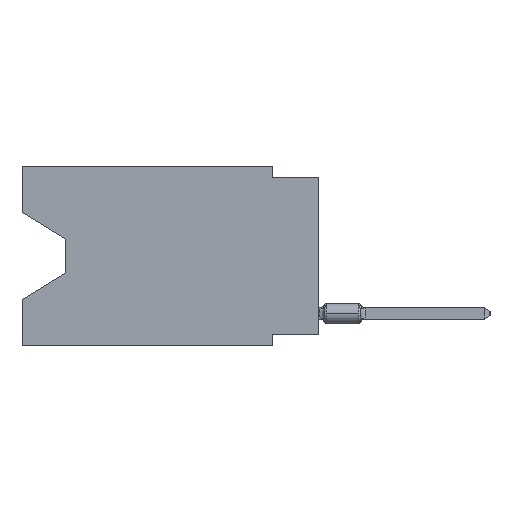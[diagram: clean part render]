
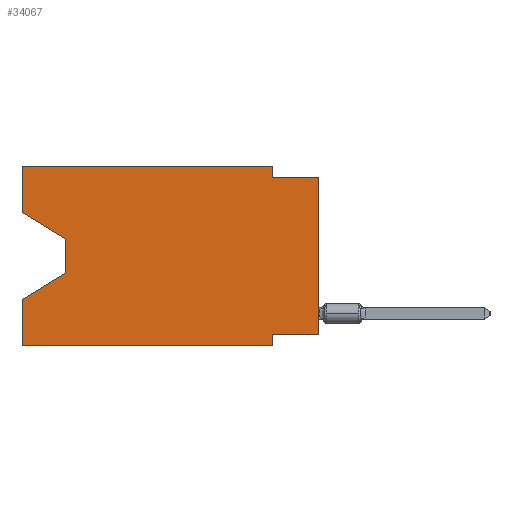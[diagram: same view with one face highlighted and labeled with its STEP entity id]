
A CAD part, left-side view. The second image highlights one B-rep face of the part: STEP entity #34067.
In plain terms, the highlighted planar face has unit normal (-1, 0, 0).
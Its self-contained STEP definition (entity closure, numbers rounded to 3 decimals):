
#341 = CARTESIAN_POINT ( 'NONE',  ( 0., 16.383, 0. ) ) ;
#2857 = VERTEX_POINT ( 'NONE', #56758 ) ;
#2975 = LINE ( 'NONE', #12578, #54716 ) ;
#3902 = EDGE_CURVE ( 'NONE', #28323, #19937, #15991, .T. ) ;
#4091 = VECTOR ( 'NONE', #23938, 1000. ) ;
#5462 = EDGE_LOOP ( 'NONE', ( #20016, #48568, #43204, #35064, #43804, #45411, #26616, #43219, #18608, #10284, #35408, #28965 ) ) ;
#6916 = DIRECTION ( 'NONE',  ( 0., -1., 0. ) ) ;
#7569 = EDGE_CURVE ( 'NONE', #16892, #58796, #11998, .T. ) ;
#8232 = LINE ( 'NONE', #8831, #47991 ) ;
#8831 = CARTESIAN_POINT ( 'NONE',  ( 0., 16.383, -2.546 ) ) ;
#8858 = LINE ( 'NONE', #13652, #53757 ) ;
#9157 = DIRECTION ( 'NONE',  ( 0., 1., 0. ) ) ;
#9626 = VECTOR ( 'NONE', #43007, 1000. ) ;
#9938 = VECTOR ( 'NONE', #54385, 1000. ) ;
#10284 = ORIENTED_EDGE ( 'NONE', *, *, #39386, .F. ) ;
#11489 = VERTEX_POINT ( 'NONE', #53122 ) ;
#11900 = AXIS2_PLACEMENT_3D ( 'NONE', #51423, #15088, #56220 ) ;
#11998 = LINE ( 'NONE', #39017, #59221 ) ;
#12578 = CARTESIAN_POINT ( 'NONE',  ( 0., 2.54, 0. ) ) ;
#13057 = EDGE_CURVE ( 'NONE', #14028, #57808, #24695, .T. ) ;
#13363 = PLANE ( 'NONE',  #11900 ) ;
#13652 = CARTESIAN_POINT ( 'NONE',  ( 0., 0., -9.271 ) ) ;
#14028 = VERTEX_POINT ( 'NONE', #24989 ) ;
#15088 = DIRECTION ( 'NONE',  ( 1., 0., 0. ) ) ;
#15991 = LINE ( 'NONE', #24410, #54266 ) ;
#16892 = VERTEX_POINT ( 'NONE', #21112 ) ;
#18530 = CARTESIAN_POINT ( 'NONE',  ( 0., 13.97, -4.013 ) ) ;
#18608 = ORIENTED_EDGE ( 'NONE', *, *, #43562, .F. ) ;
#18728 = VECTOR ( 'NONE', #57833, 1000. ) ;
#18754 = LINE ( 'NONE', #41259, #20268 ) ;
#19878 = FACE_OUTER_BOUND ( 'NONE', #5462, .T. ) ;
#19937 = VERTEX_POINT ( 'NONE', #52749 ) ;
#20016 = ORIENTED_EDGE ( 'NONE', *, *, #39729, .T. ) ;
#20268 = VECTOR ( 'NONE', #54782, 1000. ) ;
#20904 = LINE ( 'NONE', #44894, #18728 ) ;
#21112 = CARTESIAN_POINT ( 'NONE',  ( 0., 2.54, -9.271 ) ) ;
#21881 = EDGE_CURVE ( 'NONE', #57808, #56431, #39000, .T. ) ;
#22502 = EDGE_CURVE ( 'NONE', #11489, #47193, #20904, .T. ) ;
#23938 = DIRECTION ( 'NONE',  ( 0., -1., 0. ) ) ;
#24370 = CARTESIAN_POINT ( 'NONE',  ( 0., 0., -0.635 ) ) ;
#24410 = CARTESIAN_POINT ( 'NONE',  ( 0., 13.97, -4.013 ) ) ;
#24622 = CARTESIAN_POINT ( 'NONE',  ( 0., 16.383, 0. ) ) ;
#24695 = LINE ( 'NONE', #48091, #9626 ) ;
#24989 = CARTESIAN_POINT ( 'NONE',  ( 0., 16.383, -2.546 ) ) ;
#26616 = ORIENTED_EDGE ( 'NONE', *, *, #46682, .F. ) ;
#27849 = LINE ( 'NONE', #32967, #4091 ) ;
#28323 = VERTEX_POINT ( 'NONE', #18530 ) ;
#28965 = ORIENTED_EDGE ( 'NONE', *, *, #13057, .F. ) ;
#29126 = DIRECTION ( 'NONE',  ( 0., -1., 0. ) ) ;
#31140 = VECTOR ( 'NONE', #29126, 1000. ) ;
#31869 = VECTOR ( 'NONE', #6916, 1000. ) ;
#32967 = CARTESIAN_POINT ( 'NONE',  ( 0., 16.383, -9.906 ) ) ;
#34067 = ADVANCED_FACE ( 'NONE', ( #19878 ), #13363, .F. ) ;
#34291 = DIRECTION ( 'NONE',  ( 0., 0., -1. ) ) ;
#35064 = ORIENTED_EDGE ( 'NONE', *, *, #48943, .F. ) ;
#35100 = DIRECTION ( 'NONE',  ( 0., 0., -1. ) ) ;
#35408 = ORIENTED_EDGE ( 'NONE', *, *, #21881, .F. ) ;
#39000 = LINE ( 'NONE', #24622, #31140 ) ;
#39017 = CARTESIAN_POINT ( 'NONE',  ( 0., 2.54, -9.906 ) ) ;
#39386 = EDGE_CURVE ( 'NONE', #56431, #53989, #2975, .T. ) ;
#39729 = EDGE_CURVE ( 'NONE', #14028, #28323, #8232, .T. ) ;
#39842 = CARTESIAN_POINT ( 'NONE',  ( 0., 2.54, -9.906 ) ) ;
#40030 = DIRECTION ( 'NONE',  ( 0., -0.855, -0.519 ) ) ;
#40871 = LINE ( 'NONE', #341, #9938 ) ;
#41259 = CARTESIAN_POINT ( 'NONE',  ( 0., 13.97, -5.893 ) ) ;
#43007 = DIRECTION ( 'NONE',  ( 0., 0., 1. ) ) ;
#43204 = ORIENTED_EDGE ( 'NONE', *, *, #46677, .T. ) ;
#43219 = ORIENTED_EDGE ( 'NONE', *, *, #22502, .T. ) ;
#43562 = EDGE_CURVE ( 'NONE', #53989, #47193, #52840, .T. ) ;
#43680 = EDGE_CURVE ( 'NONE', #48639, #58796, #27849, .T. ) ;
#43804 = ORIENTED_EDGE ( 'NONE', *, *, #43680, .T. ) ;
#44894 = CARTESIAN_POINT ( 'NONE',  ( 0., 0., 0. ) ) ;
#45411 = ORIENTED_EDGE ( 'NONE', *, *, #7569, .F. ) ;
#46677 = EDGE_CURVE ( 'NONE', #19937, #2857, #18754, .T. ) ;
#46682 = EDGE_CURVE ( 'NONE', #11489, #16892, #8858, .T. ) ;
#47193 = VERTEX_POINT ( 'NONE', #24370 ) ;
#47467 = CARTESIAN_POINT ( 'NONE',  ( 0., 0., -0.635 ) ) ;
#47991 = VECTOR ( 'NONE', #40030, 1000. ) ;
#48091 = CARTESIAN_POINT ( 'NONE',  ( 0., 16.383, 0. ) ) ;
#48126 = CARTESIAN_POINT ( 'NONE',  ( 0., 16.383, 0. ) ) ;
#48325 = DIRECTION ( 'NONE',  ( 0., 0., -1. ) ) ;
#48568 = ORIENTED_EDGE ( 'NONE', *, *, #3902, .T. ) ;
#48639 = VERTEX_POINT ( 'NONE', #55722 ) ;
#48943 = EDGE_CURVE ( 'NONE', #48639, #2857, #40871, .T. ) ;
#50262 = CARTESIAN_POINT ( 'NONE',  ( 0., 2.54, 0. ) ) ;
#51423 = CARTESIAN_POINT ( 'NONE',  ( 0., 16.383, 0. ) ) ;
#52749 = CARTESIAN_POINT ( 'NONE',  ( 0., 13.97, -5.893 ) ) ;
#52840 = LINE ( 'NONE', #47467, #31869 ) ;
#53122 = CARTESIAN_POINT ( 'NONE',  ( 0., 0., -9.271 ) ) ;
#53757 = VECTOR ( 'NONE', #9157, 1000. ) ;
#53989 = VERTEX_POINT ( 'NONE', #59318 ) ;
#54266 = VECTOR ( 'NONE', #34291, 1000. ) ;
#54385 = DIRECTION ( 'NONE',  ( 0., 0., 1. ) ) ;
#54716 = VECTOR ( 'NONE', #35100, 1000. ) ;
#54782 = DIRECTION ( 'NONE',  ( 0., 0.855, -0.519 ) ) ;
#55722 = CARTESIAN_POINT ( 'NONE',  ( 0., 16.383, -9.906 ) ) ;
#56220 = DIRECTION ( 'NONE',  ( 0., 0., -1. ) ) ;
#56431 = VERTEX_POINT ( 'NONE', #50262 ) ;
#56758 = CARTESIAN_POINT ( 'NONE',  ( 0., 16.383, -7.36 ) ) ;
#57808 = VERTEX_POINT ( 'NONE', #48126 ) ;
#57833 = DIRECTION ( 'NONE',  ( 0., 0., 1. ) ) ;
#58796 = VERTEX_POINT ( 'NONE', #39842 ) ;
#59221 = VECTOR ( 'NONE', #48325, 1000. ) ;
#59318 = CARTESIAN_POINT ( 'NONE',  ( 0., 2.54, -0.635 ) ) ;
